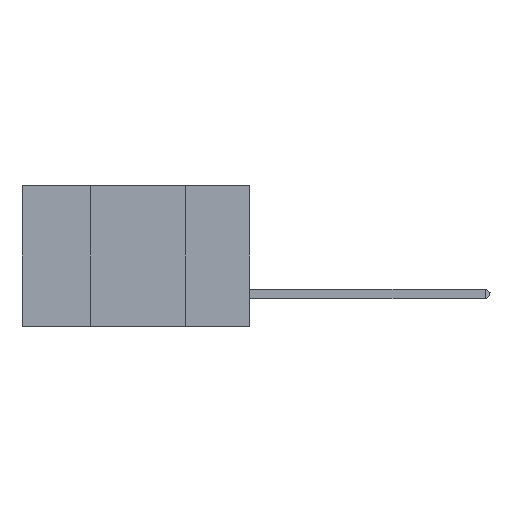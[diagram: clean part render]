
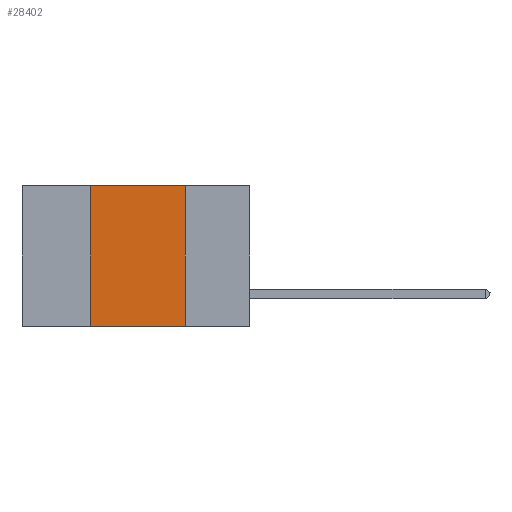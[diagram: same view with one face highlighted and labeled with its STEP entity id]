
A CAD part, left-side view. The second image highlights one B-rep face of the part: STEP entity #28402.
In plain terms, the highlighted planar face has unit normal (-1, 0, 0).
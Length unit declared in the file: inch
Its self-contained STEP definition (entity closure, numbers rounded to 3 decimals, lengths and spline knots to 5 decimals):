
#12 = EDGE_CURVE ( 'NONE', #8542, #23497, #13415, .T. ) ;
#251 = DIRECTION ( 'NONE',  ( 0., -1., 0. ) ) ;
#2453 = LINE ( 'NONE', #14766, #28189 ) ;
#3015 = VECTOR ( 'NONE', #34289, 39.37008 ) ;
#3926 = AXIS2_PLACEMENT_3D ( 'NONE', #9710, #3927, #14780 ) ;
#3927 = DIRECTION ( 'NONE',  ( 1., 0., 0. ) ) ;
#4223 = DIRECTION ( 'NONE',  ( 0., 0., -1. ) ) ;
#4579 = ORIENTED_EDGE ( 'NONE', *, *, #33969, .F. ) ;
#4629 = EDGE_LOOP ( 'NONE', ( #4579, #17749, #17099, #26235 ) ) ;
#8342 = VECTOR ( 'NONE', #11251, 39.37008 ) ;
#8542 = VERTEX_POINT ( 'NONE', #28109 ) ;
#9355 = PLANE ( 'NONE',  #3926 ) ;
#9710 = CARTESIAN_POINT ( 'NONE',  ( 0., 0.6, 0. ) ) ;
#11251 = DIRECTION ( 'NONE',  ( 0., 0., 1. ) ) ;
#13415 = LINE ( 'NONE', #29923, #8342 ) ;
#14360 = CARTESIAN_POINT ( 'NONE',  ( 0., 0.42, 0. ) ) ;
#14766 = CARTESIAN_POINT ( 'NONE',  ( 0., 0.6, 0. ) ) ;
#14780 = DIRECTION ( 'NONE',  ( 0., 0., -1. ) ) ;
#14804 = CARTESIAN_POINT ( 'NONE',  ( 0., 0.17, 0. ) ) ;
#17099 = ORIENTED_EDGE ( 'NONE', *, *, #12, .F. ) ;
#17355 = EDGE_CURVE ( 'NONE', #23497, #25028, #2453, .T. ) ;
#17749 = ORIENTED_EDGE ( 'NONE', *, *, #17355, .F. ) ;
#20259 = CARTESIAN_POINT ( 'NONE',  ( 0., 0.17, 0. ) ) ;
#20331 = FACE_OUTER_BOUND ( 'NONE', #4629, .T. ) ;
#20893 = EDGE_CURVE ( 'NONE', #8542, #29156, #24568, .T. ) ;
#23078 = VECTOR ( 'NONE', #4223, 39.37008 ) ;
#23497 = VERTEX_POINT ( 'NONE', #14360 ) ;
#24568 = LINE ( 'NONE', #29051, #3015 ) ;
#25028 = VERTEX_POINT ( 'NONE', #14804 ) ;
#26235 = ORIENTED_EDGE ( 'NONE', *, *, #20893, .T. ) ;
#28109 = CARTESIAN_POINT ( 'NONE',  ( 0., 0.42, -0.37 ) ) ;
#28189 = VECTOR ( 'NONE', #251, 39.37008 ) ;
#28402 = ADVANCED_FACE ( 'NONE', ( #20331 ), #9355, .F. ) ;
#29051 = CARTESIAN_POINT ( 'NONE',  ( 0., 0.6, -0.37 ) ) ;
#29156 = VERTEX_POINT ( 'NONE', #34042 ) ;
#29923 = CARTESIAN_POINT ( 'NONE',  ( 0., 0.42, 0. ) ) ;
#32758 = LINE ( 'NONE', #20259, #23078 ) ;
#33969 = EDGE_CURVE ( 'NONE', #25028, #29156, #32758, .T. ) ;
#34042 = CARTESIAN_POINT ( 'NONE',  ( 0., 0.17, -0.37 ) ) ;
#34289 = DIRECTION ( 'NONE',  ( 0., -1., 0. ) ) ;
